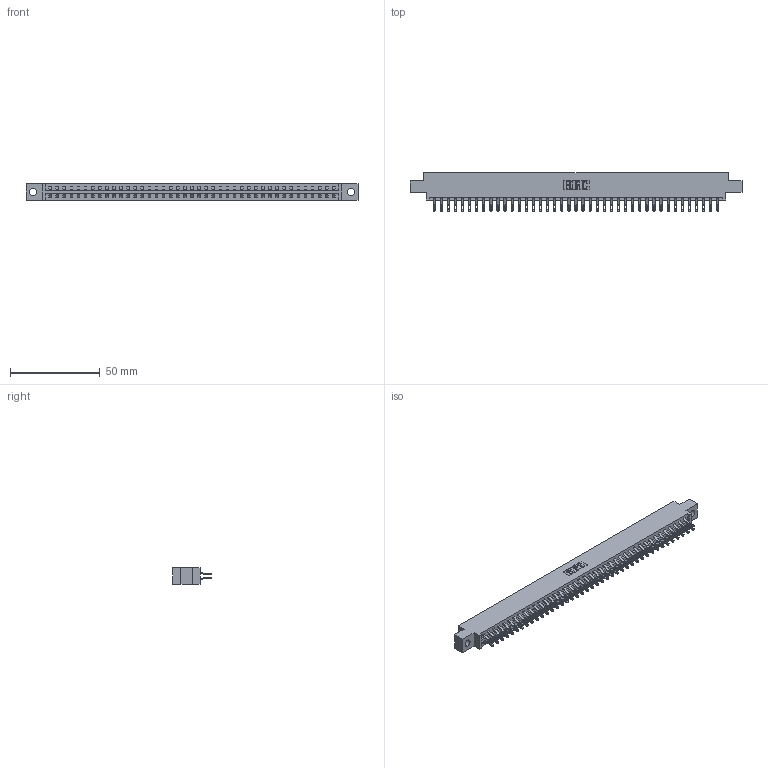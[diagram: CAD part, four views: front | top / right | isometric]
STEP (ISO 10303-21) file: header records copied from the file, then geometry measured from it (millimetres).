
FILE_DESCRIPTION (( 'STEP AP203' ), '1' );
FILE_NAME ('337-082-555-804.STEP', '2018-08-12T20:52:52', ( '' ), ( '' ), 'SwSTEP 2.0', 'SolidWorks 2016', '' );
FILE_SCHEMA (( 'CONFIG_CONTROL_DESIGN' ));
Length unit declared in the file: inch
Products named in the file (3): 337 Part_0.170 Offset - 0.156 Dia-TH; 345-292-001_555 Tail; 337-082-555-804
Assembly tree (83 placements, depth 2):
  337-082-555-804
    337 Part_0.170 Offset - 0.156 Dia-TH
    345-292-001_555 Tail  x82
Bounding box: 185.47 x 21.47 x 9.4 mm (x, y, z)
Volume: 19565.6 mm3; surface area: 22910.7 mm2
Topology: 83 solids, 83 shells, 5038 faces, 15821 edges, 10546 vertices
Faces by surface type: plane 3026, cylinder 2012
Entity records: 32379 total; most frequent: CARTESIAN_POINT 5492, ORIENTED_EDGE 5398, DIRECTION 4643, EDGE_CURVE 2699, VECTOR 2551, LINE 2551, VERTEX_POINT 1798, AXIS2_PLACEMENT_3D 1046
